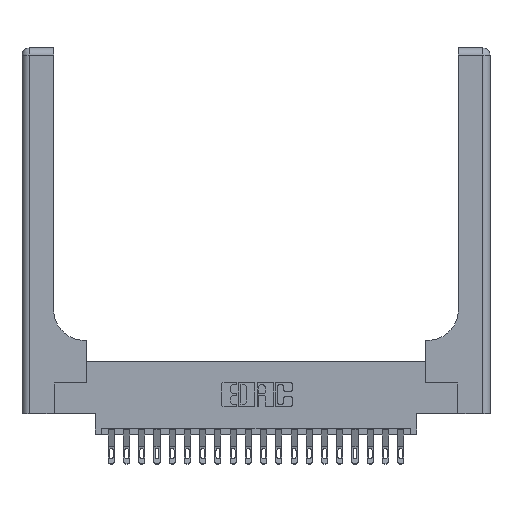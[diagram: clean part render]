
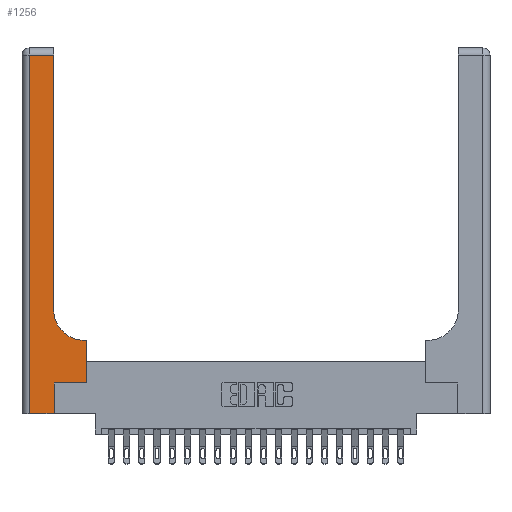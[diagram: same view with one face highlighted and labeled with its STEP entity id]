
A CAD part, top view. The second image highlights one B-rep face of the part: STEP entity #1256.
In plain terms, the highlighted planar face has unit normal (0, 0, 1).
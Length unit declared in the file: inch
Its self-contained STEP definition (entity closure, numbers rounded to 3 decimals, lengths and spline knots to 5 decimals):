
#572 = DIRECTION ( 'NONE',  ( 1., 0., 0. ) ) ;
#1236 = VECTOR ( 'NONE', #16128, 39.37008 ) ;
#1256 = ADVANCED_FACE ( 'NONE', ( #2120 ), #12300, .F. ) ;
#1525 = LINE ( 'NONE', #8538, #6173 ) ;
#1545 = VECTOR ( 'NONE', #2513, 39.37008 ) ;
#1896 = ORIENTED_EDGE ( 'NONE', *, *, #12929, .T. ) ;
#1908 = CARTESIAN_POINT ( 'NONE',  ( 0.51, 0.6, 0.37 ) ) ;
#2120 = FACE_OUTER_BOUND ( 'NONE', #10892, .T. ) ;
#2310 = VERTEX_POINT ( 'NONE', #4372 ) ;
#2513 = DIRECTION ( 'NONE',  ( -1., 0., 0. ) ) ;
#2927 = CARTESIAN_POINT ( 'NONE',  ( 0.26, 3., 0.37 ) ) ;
#2986 = ORIENTED_EDGE ( 'NONE', *, *, #7750, .T. ) ;
#3520 = LINE ( 'NONE', #13489, #15212 ) ;
#4222 = ORIENTED_EDGE ( 'NONE', *, *, #16557, .T. ) ;
#4372 = CARTESIAN_POINT ( 'NONE',  ( 0.265, 0., 0.37 ) ) ;
#4527 = LINE ( 'NONE', #19861, #1545 ) ;
#4572 = VECTOR ( 'NONE', #5556, 39.37008 ) ;
#4681 = VERTEX_POINT ( 'NONE', #20216 ) ;
#4770 = AXIS2_PLACEMENT_3D ( 'NONE', #8915, #20806, #15452 ) ;
#4796 = DIRECTION ( 'NONE',  ( 1., 0., 0. ) ) ;
#5076 = CARTESIAN_POINT ( 'NONE',  ( 0.06, 0., 0.37 ) ) ;
#5275 = LINE ( 'NONE', #19036, #1236 ) ;
#5556 = DIRECTION ( 'NONE',  ( 0., 1., 0. ) ) ;
#6173 = VECTOR ( 'NONE', #16754, 39.37008 ) ;
#6759 = DIRECTION ( 'NONE',  ( -1., 0., 0. ) ) ;
#7671 = VECTOR ( 'NONE', #14888, 39.37008 ) ;
#7750 = EDGE_CURVE ( 'NONE', #14465, #21400, #13411, .T. ) ;
#7806 = AXIS2_PLACEMENT_3D ( 'NONE', #14110, #12867, #572 ) ;
#7977 = ORIENTED_EDGE ( 'NONE', *, *, #8607, .T. ) ;
#7993 = VECTOR ( 'NONE', #13442, 39.37008 ) ;
#8240 = EDGE_CURVE ( 'NONE', #17691, #2310, #1525, .T. ) ;
#8538 = CARTESIAN_POINT ( 'NONE',  ( 0., 0., 0.37 ) ) ;
#8607 = EDGE_CURVE ( 'NONE', #11970, #14392, #4527, .T. ) ;
#8915 = CARTESIAN_POINT ( 'NONE',  ( 0., 3., 0.37 ) ) ;
#9325 = ORIENTED_EDGE ( 'NONE', *, *, #18130, .T. ) ;
#10377 = EDGE_CURVE ( 'NONE', #10996, #4681, #20165, .T. ) ;
#10412 = VECTOR ( 'NONE', #4796, 39.37008 ) ;
#10590 = EDGE_CURVE ( 'NONE', #13096, #17691, #5275, .T. ) ;
#10892 = EDGE_LOOP ( 'NONE', ( #12771, #11321, #13280, #16518, #1896, #2986, #4222, #7977, #9325 ) ) ;
#10996 = VERTEX_POINT ( 'NONE', #13632 ) ;
#11321 = ORIENTED_EDGE ( 'NONE', *, *, #13412, .T. ) ;
#11970 = VERTEX_POINT ( 'NONE', #21518 ) ;
#12060 = CARTESIAN_POINT ( 'NONE',  ( 0.06, 2.94, 0.37 ) ) ;
#12300 = PLANE ( 'NONE',  #4770 ) ;
#12771 = ORIENTED_EDGE ( 'NONE', *, *, #10377, .T. ) ;
#12867 = DIRECTION ( 'NONE',  ( 0., 0., -1. ) ) ;
#12929 = EDGE_CURVE ( 'NONE', #2310, #14465, #18350, .T. ) ;
#13096 = VERTEX_POINT ( 'NONE', #12060 ) ;
#13280 = ORIENTED_EDGE ( 'NONE', *, *, #10590, .T. ) ;
#13411 = LINE ( 'NONE', #20461, #10412 ) ;
#13412 = EDGE_CURVE ( 'NONE', #4681, #13096, #3520, .T. ) ;
#13442 = DIRECTION ( 'NONE',  ( 0., 1., 0. ) ) ;
#13489 = CARTESIAN_POINT ( 'NONE',  ( 0., 2.94, 0.37 ) ) ;
#13632 = CARTESIAN_POINT ( 'NONE',  ( 0.26, 0.85, 0.37 ) ) ;
#14053 = LINE ( 'NONE', #17201, #4572 ) ;
#14110 = CARTESIAN_POINT ( 'NONE',  ( 0.51, 0.85, 0.37 ) ) ;
#14339 = CARTESIAN_POINT ( 'NONE',  ( 0.528, 0.25, 0.37 ) ) ;
#14392 = VERTEX_POINT ( 'NONE', #1908 ) ;
#14465 = VERTEX_POINT ( 'NONE', #18922 ) ;
#14888 = DIRECTION ( 'NONE',  ( 0., 1., 0. ) ) ;
#15212 = VECTOR ( 'NONE', #6759, 39.37008 ) ;
#15452 = DIRECTION ( 'NONE',  ( -1., 0., 0. ) ) ;
#16128 = DIRECTION ( 'NONE',  ( 0., -1., 0. ) ) ;
#16518 = ORIENTED_EDGE ( 'NONE', *, *, #8240, .T. ) ;
#16557 = EDGE_CURVE ( 'NONE', #21400, #11970, #14053, .T. ) ;
#16754 = DIRECTION ( 'NONE',  ( 1., 0., 0. ) ) ;
#17201 = CARTESIAN_POINT ( 'NONE',  ( 0.528, 0.25, 0.37 ) ) ;
#17496 = CIRCLE ( 'NONE', #7806, 0.25 ) ;
#17691 = VERTEX_POINT ( 'NONE', #5076 ) ;
#18130 = EDGE_CURVE ( 'NONE', #14392, #10996, #17496, .T. ) ;
#18350 = LINE ( 'NONE', #20133, #7671 ) ;
#18922 = CARTESIAN_POINT ( 'NONE',  ( 0.265, 0.25, 0.37 ) ) ;
#19036 = CARTESIAN_POINT ( 'NONE',  ( 0.06, 3., 0.37 ) ) ;
#19861 = CARTESIAN_POINT ( 'NONE',  ( 0.26, 0.6, 0.37 ) ) ;
#20133 = CARTESIAN_POINT ( 'NONE',  ( 0.265, 0., 0.37 ) ) ;
#20165 = LINE ( 'NONE', #2927, #7993 ) ;
#20216 = CARTESIAN_POINT ( 'NONE',  ( 0.26, 2.94, 0.37 ) ) ;
#20461 = CARTESIAN_POINT ( 'NONE',  ( 0.265, 0.25, 0.37 ) ) ;
#20806 = DIRECTION ( 'NONE',  ( 0., 0., -1. ) ) ;
#21400 = VERTEX_POINT ( 'NONE', #14339 ) ;
#21518 = CARTESIAN_POINT ( 'NONE',  ( 0.528, 0.6, 0.37 ) ) ;
